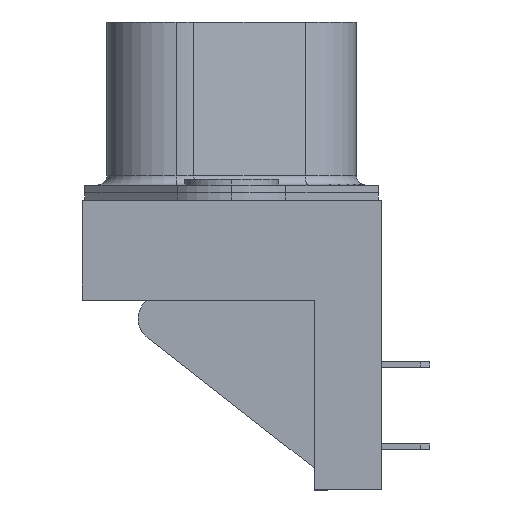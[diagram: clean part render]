
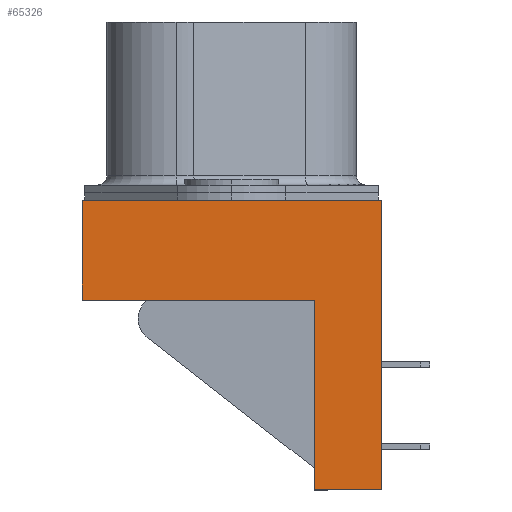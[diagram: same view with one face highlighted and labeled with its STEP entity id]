
A CAD part, left-side view. The second image highlights one B-rep face of the part: STEP entity #65326.
In plain terms, the highlighted planar face has unit normal (-1, 0, 0).
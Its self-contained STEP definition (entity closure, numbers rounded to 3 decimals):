
#3804 = DIRECTION ( 'NONE',  ( -1., 0., 0. ) ) ;
#8767 = CARTESIAN_POINT ( 'NONE',  ( -4.125, -4.3, -15.1 ) ) ;
#9649 = CARTESIAN_POINT ( 'NONE',  ( -4.125, -4.3, -15.1 ) ) ;
#14814 = ORIENTED_EDGE ( 'NONE', *, *, #170247, .F. ) ;
#20851 = CARTESIAN_POINT ( 'NONE',  ( -4.125, 7.8, -5.2 ) ) ;
#21314 = LINE ( 'NONE', #8767, #96129 ) ;
#26614 = ORIENTED_EDGE ( 'NONE', *, *, #47272, .T. ) ;
#32826 = VERTEX_POINT ( 'NONE', #153885 ) ;
#33957 = DIRECTION ( 'NONE',  ( 0., -1., 0. ) ) ;
#35183 = EDGE_CURVE ( 'NONE', #149784, #32826, #91306, .T. ) ;
#36830 = EDGE_CURVE ( 'NONE', #32826, #68229, #102145, .T. ) ;
#39708 = VECTOR ( 'NONE', #33957, 1000. ) ;
#42084 = VECTOR ( 'NONE', #100301, 1000. ) ;
#47272 = EDGE_CURVE ( 'NONE', #85859, #77085, #71637, .T. ) ;
#53041 = VERTEX_POINT ( 'NONE', #115959 ) ;
#53292 = ORIENTED_EDGE ( 'NONE', *, *, #36830, .F. ) ;
#58525 = DIRECTION ( 'NONE',  ( 0., -1., 0. ) ) ;
#59068 = CARTESIAN_POINT ( 'NONE',  ( -4.125, 7.8, -15.1 ) ) ;
#65280 = CARTESIAN_POINT ( 'NONE',  ( -4.125, 7.8, -15.1 ) ) ;
#65326 = ADVANCED_FACE ( 'NONE', ( #71965 ), #126650, .T. ) ;
#65822 = ORIENTED_EDGE ( 'NONE', *, *, #35183, .F. ) ;
#67887 = CARTESIAN_POINT ( 'NONE',  ( -4.125, 7.8, -5.2 ) ) ;
#68229 = VERTEX_POINT ( 'NONE', #158222 ) ;
#70610 = EDGE_CURVE ( 'NONE', #77085, #68229, #100849, .T. ) ;
#71637 = LINE ( 'NONE', #59068, #42084 ) ;
#71965 = FACE_OUTER_BOUND ( 'NONE', #77167, .T. ) ;
#74158 = VECTOR ( 'NONE', #134289, 1000. ) ;
#77085 = VERTEX_POINT ( 'NONE', #155275 ) ;
#77167 = EDGE_LOOP ( 'NONE', ( #14814, #141200, #26614, #142355, #53292, #65822 ) ) ;
#85859 = VERTEX_POINT ( 'NONE', #9649 ) ;
#91306 = LINE ( 'NONE', #65280, #74158 ) ;
#96129 = VECTOR ( 'NONE', #120795, 1000. ) ;
#100301 = DIRECTION ( 'NONE',  ( 0., -1., 0. ) ) ;
#100849 = LINE ( 'NONE', #103497, #148741 ) ;
#102145 = LINE ( 'NONE', #156804, #39708 ) ;
#103497 = CARTESIAN_POINT ( 'NONE',  ( -4.125, -7.8, -15.1 ) ) ;
#105575 = DIRECTION ( 'NONE',  ( 0., 1., 0. ) ) ;
#107361 = LINE ( 'NONE', #67887, #139153 ) ;
#113198 = CARTESIAN_POINT ( 'NONE',  ( -4.125, 7.8, -15.1 ) ) ;
#115959 = CARTESIAN_POINT ( 'NONE',  ( -4.125, -4.3, -5.2 ) ) ;
#120795 = DIRECTION ( 'NONE',  ( 0., 0., 1. ) ) ;
#126650 = PLANE ( 'NONE',  #168480 ) ;
#134289 = DIRECTION ( 'NONE',  ( 0., 0., 1. ) ) ;
#139153 = VECTOR ( 'NONE', #105575, 1000. ) ;
#141200 = ORIENTED_EDGE ( 'NONE', *, *, #158635, .F. ) ;
#142355 = ORIENTED_EDGE ( 'NONE', *, *, #70610, .T. ) ;
#142933 = DIRECTION ( 'NONE',  ( 0., 0., 1. ) ) ;
#148741 = VECTOR ( 'NONE', #142933, 1000. ) ;
#149784 = VERTEX_POINT ( 'NONE', #20851 ) ;
#153885 = CARTESIAN_POINT ( 'NONE',  ( -4.125, 7.8, 0. ) ) ;
#155275 = CARTESIAN_POINT ( 'NONE',  ( -4.125, -7.8, -15.1 ) ) ;
#156804 = CARTESIAN_POINT ( 'NONE',  ( -4.125, 7.8, 0. ) ) ;
#158222 = CARTESIAN_POINT ( 'NONE',  ( -4.125, -7.8, 0. ) ) ;
#158635 = EDGE_CURVE ( 'NONE', #85859, #53041, #21314, .T. ) ;
#168480 = AXIS2_PLACEMENT_3D ( 'NONE', #113198, #3804, #58525 ) ;
#170247 = EDGE_CURVE ( 'NONE', #53041, #149784, #107361, .T. ) ;
